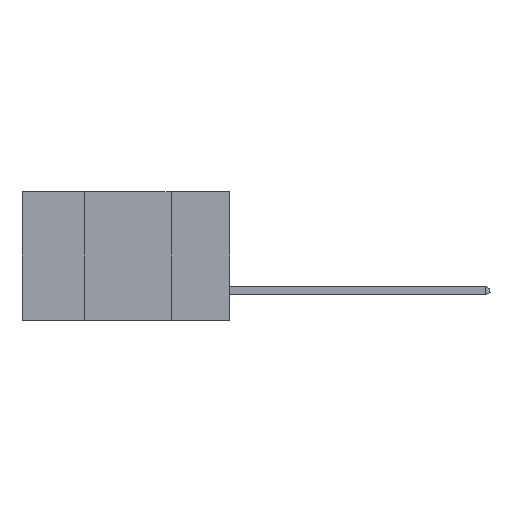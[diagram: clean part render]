
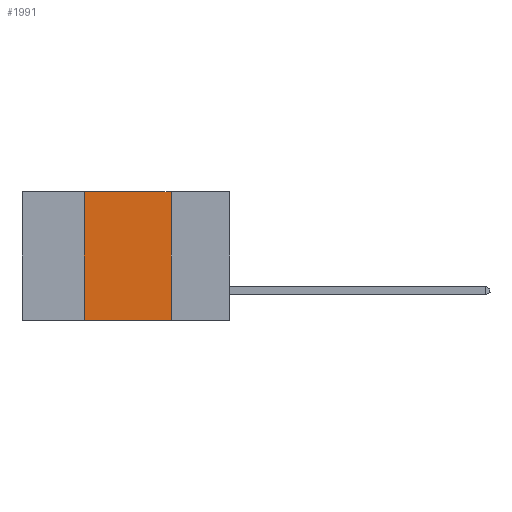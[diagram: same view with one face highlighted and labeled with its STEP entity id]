
A CAD part, left-side view. The second image highlights one B-rep face of the part: STEP entity #1991.
In plain terms, the highlighted planar face has unit normal (-1, 0, 0).
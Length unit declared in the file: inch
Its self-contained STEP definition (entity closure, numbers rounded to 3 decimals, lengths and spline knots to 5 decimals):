
#1752 = FACE_OUTER_BOUND ( 'NONE', #15058, .T. ) ;
#1991 = ADVANCED_FACE ( 'NONE', ( #1752 ), #8215, .F. ) ;
#2072 = CARTESIAN_POINT ( 'NONE',  ( 0., 0.6, 0. ) ) ;
#2438 = LINE ( 'NONE', #4124, #7286 ) ;
#2902 = VERTEX_POINT ( 'NONE', #3880 ) ;
#2930 = VERTEX_POINT ( 'NONE', #7605 ) ;
#3880 = CARTESIAN_POINT ( 'NONE',  ( 0., 0.17, 0. ) ) ;
#4124 = CARTESIAN_POINT ( 'NONE',  ( 0., 0.6, 0. ) ) ;
#4280 = DIRECTION ( 'NONE',  ( 0., -1., 0. ) ) ;
#4391 = VERTEX_POINT ( 'NONE', #8695 ) ;
#5355 = VECTOR ( 'NONE', #11035, 39.37008 ) ;
#6626 = ORIENTED_EDGE ( 'NONE', *, *, #7982, .F. ) ;
#7102 = EDGE_CURVE ( 'NONE', #2930, #2902, #2438, .T. ) ;
#7171 = DIRECTION ( 'NONE',  ( 1., 0., 0. ) ) ;
#7286 = VECTOR ( 'NONE', #12701, 39.37008 ) ;
#7333 = VECTOR ( 'NONE', #4280, 39.37008 ) ;
#7605 = CARTESIAN_POINT ( 'NONE',  ( 0., 0.42, 0. ) ) ;
#7982 = EDGE_CURVE ( 'NONE', #2902, #4391, #13798, .T. ) ;
#8149 = ORIENTED_EDGE ( 'NONE', *, *, #13001, .F. ) ;
#8215 = PLANE ( 'NONE',  #8867 ) ;
#8695 = CARTESIAN_POINT ( 'NONE',  ( 0., 0.17, -0.37 ) ) ;
#8867 = AXIS2_PLACEMENT_3D ( 'NONE', #2072, #7171, #15709 ) ;
#9633 = ORIENTED_EDGE ( 'NONE', *, *, #9884, .T. ) ;
#9691 = VECTOR ( 'NONE', #14678, 39.37008 ) ;
#9884 = EDGE_CURVE ( 'NONE', #10106, #4391, #12367, .T. ) ;
#9962 = LINE ( 'NONE', #13451, #5355 ) ;
#10106 = VERTEX_POINT ( 'NONE', #11809 ) ;
#10877 = CARTESIAN_POINT ( 'NONE',  ( 0., 0.17, 0. ) ) ;
#11035 = DIRECTION ( 'NONE',  ( 0., 0., 1. ) ) ;
#11340 = ORIENTED_EDGE ( 'NONE', *, *, #7102, .F. ) ;
#11809 = CARTESIAN_POINT ( 'NONE',  ( 0., 0.42, -0.37 ) ) ;
#12367 = LINE ( 'NONE', #14131, #7333 ) ;
#12701 = DIRECTION ( 'NONE',  ( 0., -1., 0. ) ) ;
#13001 = EDGE_CURVE ( 'NONE', #10106, #2930, #9962, .T. ) ;
#13451 = CARTESIAN_POINT ( 'NONE',  ( 0., 0.42, 0. ) ) ;
#13798 = LINE ( 'NONE', #10877, #9691 ) ;
#14131 = CARTESIAN_POINT ( 'NONE',  ( 0., 0.6, -0.37 ) ) ;
#14678 = DIRECTION ( 'NONE',  ( 0., 0., -1. ) ) ;
#15058 = EDGE_LOOP ( 'NONE', ( #6626, #11340, #8149, #9633 ) ) ;
#15709 = DIRECTION ( 'NONE',  ( 0., 0., -1. ) ) ;
